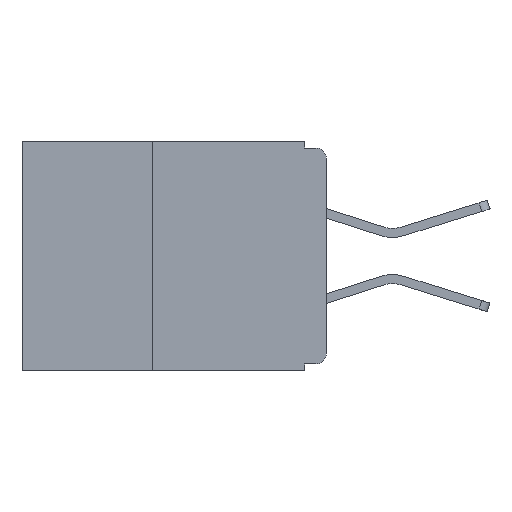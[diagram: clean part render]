
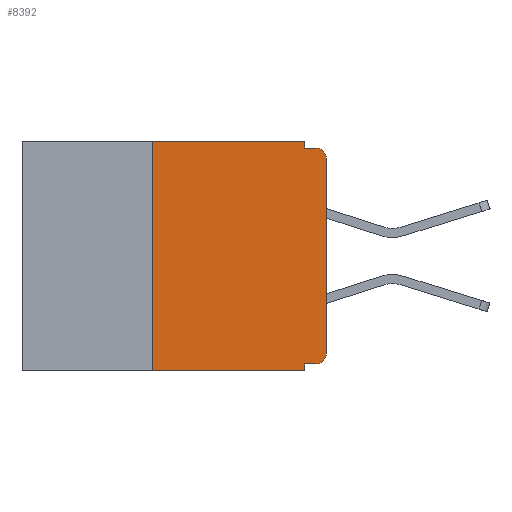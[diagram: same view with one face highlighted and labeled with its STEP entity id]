
A CAD part, left-side view. The second image highlights one B-rep face of the part: STEP entity #8392.
In plain terms, the highlighted planar face has unit normal (-1, 0, 0).
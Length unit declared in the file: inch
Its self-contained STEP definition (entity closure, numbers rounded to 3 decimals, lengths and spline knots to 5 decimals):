
#109 = EDGE_CURVE ( 'NONE', #11098, #10213, #4485, .T. ) ;
#512 = DIRECTION ( 'NONE',  ( 0., -1., 0. ) ) ;
#587 = VERTEX_POINT ( 'NONE', #23622 ) ;
#879 = CARTESIAN_POINT ( 'NONE',  ( 0., 0.437, -0.33 ) ) ;
#1218 = EDGE_CURVE ( 'NONE', #2810, #20757, #11819, .T. ) ;
#1317 = VECTOR ( 'NONE', #17082, 39.37008 ) ;
#1350 = EDGE_CURVE ( 'NONE', #15995, #10213, #17645, .T. ) ;
#1902 = VECTOR ( 'NONE', #22541, 39.37008 ) ;
#2129 = VERTEX_POINT ( 'NONE', #6487 ) ;
#2201 = ORIENTED_EDGE ( 'NONE', *, *, #9939, .F. ) ;
#2267 = AXIS2_PLACEMENT_3D ( 'NONE', #15579, #4314, #17448 ) ;
#2567 = EDGE_CURVE ( 'NONE', #15995, #2129, #18759, .T. ) ;
#2691 = VECTOR ( 'NONE', #512, 39.37008 ) ;
#2810 = VERTEX_POINT ( 'NONE', #12362 ) ;
#2868 = CIRCLE ( 'NONE', #5237, 0.015 ) ;
#3522 = CARTESIAN_POINT ( 'NONE',  ( 0., 0., -0.305 ) ) ;
#3662 = EDGE_CURVE ( 'NONE', #6386, #587, #2868, .T. ) ;
#3787 = VECTOR ( 'NONE', #6126, 39.37008 ) ;
#3808 = EDGE_CURVE ( 'NONE', #14623, #13808, #14887, .T. ) ;
#3913 = VECTOR ( 'NONE', #11794, 39.37008 ) ;
#3928 = VECTOR ( 'NONE', #9885, 39.37008 ) ;
#4138 = CARTESIAN_POINT ( 'NONE',  ( 0., 0.25, -0.33 ) ) ;
#4147 = VECTOR ( 'NONE', #12926, 39.37008 ) ;
#4211 = ORIENTED_EDGE ( 'NONE', *, *, #1350, .T. ) ;
#4314 = DIRECTION ( 'NONE',  ( 1., 0., 0. ) ) ;
#4485 = LINE ( 'NONE', #20233, #3928 ) ;
#5190 = CARTESIAN_POINT ( 'NONE',  ( 0., 0.031, -0.32 ) ) ;
#5237 = AXIS2_PLACEMENT_3D ( 'NONE', #18593, #18585, #18505 ) ;
#5819 = CARTESIAN_POINT ( 'NONE',  ( 0., 0., -0.32 ) ) ;
#6102 = PLANE ( 'NONE',  #2267 ) ;
#6126 = DIRECTION ( 'NONE',  ( 0., 0., 1. ) ) ;
#6386 = VERTEX_POINT ( 'NONE', #21922 ) ;
#6487 = CARTESIAN_POINT ( 'NONE',  ( 0., 0.25, 0. ) ) ;
#7150 = CARTESIAN_POINT ( 'NONE',  ( 0., 0.031, 0. ) ) ;
#7919 = DIRECTION ( 'NONE',  ( 0., 0., -1. ) ) ;
#8392 = ADVANCED_FACE ( 'NONE', ( #15100 ), #6102, .F. ) ;
#8411 = DIRECTION ( 'NONE',  ( 0., 0., -1. ) ) ;
#8565 = DIRECTION ( 'NONE',  ( -1., 0., 0. ) ) ;
#8615 = CARTESIAN_POINT ( 'NONE',  ( 0., 0.015, -0.305 ) ) ;
#9054 = EDGE_LOOP ( 'NONE', ( #13829, #22292, #18504, #18293, #9462, #19474, #4211, #9188, #2201, #13658 ) ) ;
#9087 = CARTESIAN_POINT ( 'NONE',  ( 0., 0.25, -0.33 ) ) ;
#9188 = ORIENTED_EDGE ( 'NONE', *, *, #109, .F. ) ;
#9462 = ORIENTED_EDGE ( 'NONE', *, *, #10496, .F. ) ;
#9724 = CARTESIAN_POINT ( 'NONE',  ( 0., 0.031, -0.01 ) ) ;
#9885 = DIRECTION ( 'NONE',  ( 0., 0., -1. ) ) ;
#9939 = EDGE_CURVE ( 'NONE', #2810, #11098, #11260, .T. ) ;
#10213 = VERTEX_POINT ( 'NONE', #14080 ) ;
#10282 = CARTESIAN_POINT ( 'NONE',  ( 0., 0.031, 0. ) ) ;
#10496 = EDGE_CURVE ( 'NONE', #2129, #14623, #24022, .T. ) ;
#10934 = CARTESIAN_POINT ( 'NONE',  ( 0., 0.437, 0. ) ) ;
#11098 = VERTEX_POINT ( 'NONE', #5190 ) ;
#11260 = LINE ( 'NONE', #5819, #1317 ) ;
#11280 = CARTESIAN_POINT ( 'NONE',  ( 0., 0., 0. ) ) ;
#11794 = DIRECTION ( 'NONE',  ( 0., -1., 0. ) ) ;
#11819 = CIRCLE ( 'NONE', #13277, 0.015 ) ;
#11877 = LINE ( 'NONE', #11280, #1902 ) ;
#12362 = CARTESIAN_POINT ( 'NONE',  ( 0., 0.015, -0.32 ) ) ;
#12926 = DIRECTION ( 'NONE',  ( 0., -1., 0. ) ) ;
#13277 = AXIS2_PLACEMENT_3D ( 'NONE', #8615, #8565, #8411 ) ;
#13658 = ORIENTED_EDGE ( 'NONE', *, *, #1218, .T. ) ;
#13808 = VERTEX_POINT ( 'NONE', #9724 ) ;
#13829 = ORIENTED_EDGE ( 'NONE', *, *, #22499, .T. ) ;
#13923 = LINE ( 'NONE', #15548, #3913 ) ;
#14080 = CARTESIAN_POINT ( 'NONE',  ( 0., 0.031, -0.33 ) ) ;
#14623 = VERTEX_POINT ( 'NONE', #10282 ) ;
#14887 = LINE ( 'NONE', #7150, #21251 ) ;
#15100 = FACE_OUTER_BOUND ( 'NONE', #9054, .T. ) ;
#15548 = CARTESIAN_POINT ( 'NONE',  ( 0., 0., -0.01 ) ) ;
#15579 = CARTESIAN_POINT ( 'NONE',  ( 0., 0.437, 0. ) ) ;
#15995 = VERTEX_POINT ( 'NONE', #9087 ) ;
#17082 = DIRECTION ( 'NONE',  ( 0., 1., 0. ) ) ;
#17448 = DIRECTION ( 'NONE',  ( 0., 0., -1. ) ) ;
#17485 = EDGE_CURVE ( 'NONE', #13808, #587, #13923, .T. ) ;
#17645 = LINE ( 'NONE', #879, #2691 ) ;
#18293 = ORIENTED_EDGE ( 'NONE', *, *, #3808, .F. ) ;
#18504 = ORIENTED_EDGE ( 'NONE', *, *, #17485, .F. ) ;
#18505 = DIRECTION ( 'NONE',  ( 0., 0., -1. ) ) ;
#18585 = DIRECTION ( 'NONE',  ( -1., 0., 0. ) ) ;
#18593 = CARTESIAN_POINT ( 'NONE',  ( 0., 0.015, -0.025 ) ) ;
#18759 = LINE ( 'NONE', #4138, #3787 ) ;
#19474 = ORIENTED_EDGE ( 'NONE', *, *, #2567, .F. ) ;
#20233 = CARTESIAN_POINT ( 'NONE',  ( 0., 0.031, -0.33 ) ) ;
#20757 = VERTEX_POINT ( 'NONE', #3522 ) ;
#21251 = VECTOR ( 'NONE', #7919, 39.37008 ) ;
#21922 = CARTESIAN_POINT ( 'NONE',  ( 0., 0., -0.025 ) ) ;
#22292 = ORIENTED_EDGE ( 'NONE', *, *, #3662, .T. ) ;
#22499 = EDGE_CURVE ( 'NONE', #20757, #6386, #11877, .T. ) ;
#22541 = DIRECTION ( 'NONE',  ( 0., 0., 1. ) ) ;
#23622 = CARTESIAN_POINT ( 'NONE',  ( 0., 0.015, -0.01 ) ) ;
#24022 = LINE ( 'NONE', #10934, #4147 ) ;
